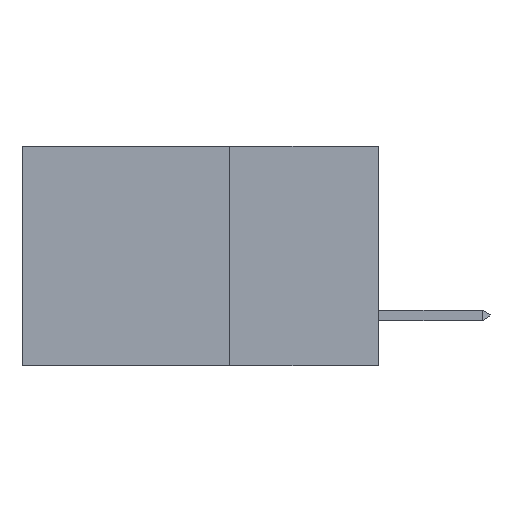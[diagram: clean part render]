
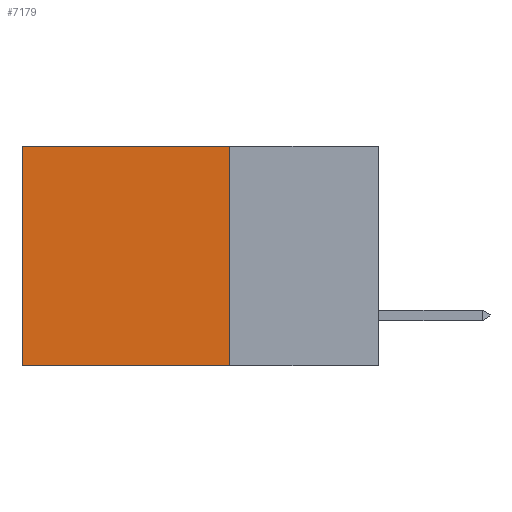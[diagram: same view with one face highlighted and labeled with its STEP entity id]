
A CAD part, left-side view. The second image highlights one B-rep face of the part: STEP entity #7179.
In plain terms, the highlighted planar face has unit normal (-1, 0, 0).
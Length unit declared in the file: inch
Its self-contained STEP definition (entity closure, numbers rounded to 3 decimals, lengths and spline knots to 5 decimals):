
#924 = EDGE_CURVE ( 'NONE', #11836, #5316, #1491, .T. ) ;
#1491 = LINE ( 'NONE', #10624, #4785 ) ;
#1636 = DIRECTION ( 'NONE',  ( 0., 0., -1. ) ) ;
#1715 = LINE ( 'NONE', #10651, #11455 ) ;
#1935 = PLANE ( 'NONE',  #11305 ) ;
#2084 = EDGE_CURVE ( 'NONE', #10172, #5316, #1715, .T. ) ;
#2294 = ORIENTED_EDGE ( 'NONE', *, *, #2084, .F. ) ;
#2689 = DIRECTION ( 'NONE',  ( 0., 0., -1. ) ) ;
#4412 = ORIENTED_EDGE ( 'NONE', *, *, #4634, .T. ) ;
#4545 = CARTESIAN_POINT ( 'NONE',  ( 0.2615, 0.25, -0.37 ) ) ;
#4580 = CARTESIAN_POINT ( 'NONE',  ( 0.2615, 0.6, 0. ) ) ;
#4606 = EDGE_LOOP ( 'NONE', ( #5640, #2294, #6374, #4412 ) ) ;
#4634 = EDGE_CURVE ( 'NONE', #4641, #11836, #7925, .T. ) ;
#4641 = VERTEX_POINT ( 'NONE', #12153 ) ;
#4785 = VECTOR ( 'NONE', #8608, 39.37008 ) ;
#5316 = VERTEX_POINT ( 'NONE', #10676 ) ;
#5570 = FACE_OUTER_BOUND ( 'NONE', #4606, .T. ) ;
#5640 = ORIENTED_EDGE ( 'NONE', *, *, #924, .T. ) ;
#6028 = CARTESIAN_POINT ( 'NONE',  ( 0.2615, 0.25, 0. ) ) ;
#6374 = ORIENTED_EDGE ( 'NONE', *, *, #6785, .F. ) ;
#6785 = EDGE_CURVE ( 'NONE', #4641, #10172, #11778, .T. ) ;
#7179 = ADVANCED_FACE ( 'NONE', ( #5570 ), #1935, .F. ) ;
#7877 = CARTESIAN_POINT ( 'NONE',  ( 0.2615, 0.25, -0.37 ) ) ;
#7925 = LINE ( 'NONE', #6028, #11805 ) ;
#8608 = DIRECTION ( 'NONE',  ( 0., 0., -1. ) ) ;
#8662 = CARTESIAN_POINT ( 'NONE',  ( 0.2615, 0.25, -0.37 ) ) ;
#9952 = VECTOR ( 'NONE', #1636, 39.37008 ) ;
#10172 = VERTEX_POINT ( 'NONE', #4545 ) ;
#10624 = CARTESIAN_POINT ( 'NONE',  ( 0.2615, 0.6, -0.37 ) ) ;
#10651 = CARTESIAN_POINT ( 'NONE',  ( 0.2615, 0.25, -0.37 ) ) ;
#10676 = CARTESIAN_POINT ( 'NONE',  ( 0.2615, 0.6, -0.37 ) ) ;
#10905 = DIRECTION ( 'NONE',  ( 0., 1., 0. ) ) ;
#11305 = AXIS2_PLACEMENT_3D ( 'NONE', #8662, #11832, #2689 ) ;
#11455 = VECTOR ( 'NONE', #10905, 39.37008 ) ;
#11778 = LINE ( 'NONE', #7877, #9952 ) ;
#11805 = VECTOR ( 'NONE', #12030, 39.37008 ) ;
#11832 = DIRECTION ( 'NONE',  ( 1., 0., 0. ) ) ;
#11836 = VERTEX_POINT ( 'NONE', #4580 ) ;
#12030 = DIRECTION ( 'NONE',  ( 0., 1., 0. ) ) ;
#12153 = CARTESIAN_POINT ( 'NONE',  ( 0.2615, 0.25, 0. ) ) ;
